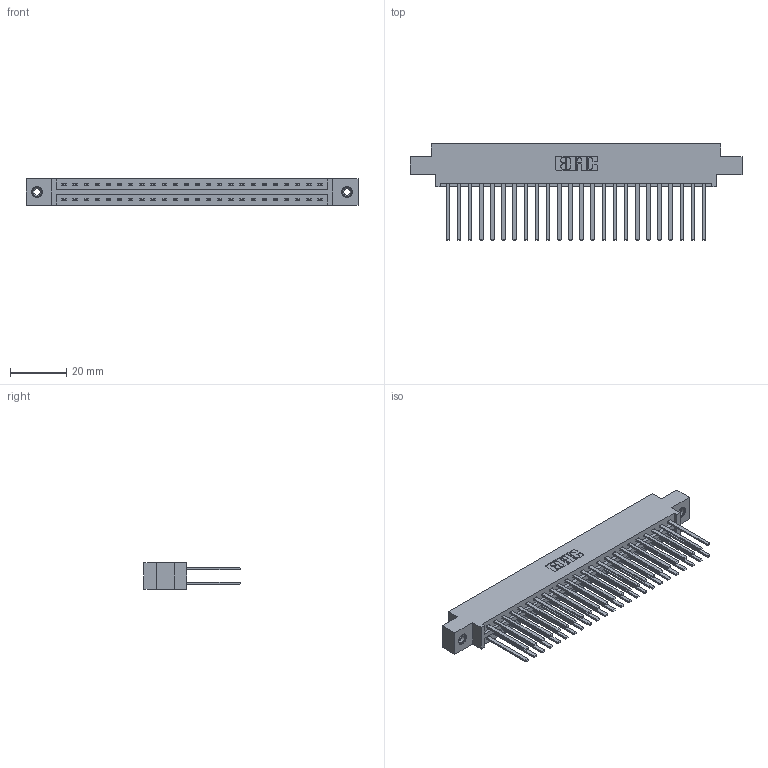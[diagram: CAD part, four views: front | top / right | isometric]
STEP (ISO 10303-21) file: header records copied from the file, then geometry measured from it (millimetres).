
FILE_DESCRIPTION (( 'STEP AP203' ), '1' );
FILE_NAME ('337-048-544-808.STEP', '2019-10-11T15:40:10', ( '' ), ( '' ), 'SwSTEP 2.0', 'SolidWorks 2016', '' );
FILE_SCHEMA (( 'CONFIG_CONTROL_DESIGN' ));
Length unit declared in the file: inch
Products named in the file (4): 345-250-001_345-250-003-102; 337-048-544-808; 337 Part_0.170 Offset - 0.156 Dia-TI; 345-292-001_345-293-144
Assembly tree (51 placements, depth 2):
  337-048-544-808
    337 Part_0.170 Offset - 0.156 Dia-TI
    345-292-001_345-293-144  x48
    345-250-001_345-250-003-102  x2
Bounding box: 118.11 x 34.3 x 9.4 mm (x, y, z)
Volume: 12756.6 mm3; surface area: 16576.4 mm2
Topology: 51 solids, 51 shells, 2482 faces, 7323 edges, 4810 vertices
Faces by surface type: plane 1738, cylinder 728, cone 12, torus 4
Entity records: 22070 total; most frequent: CARTESIAN_POINT 3713, ORIENTED_EDGE 3642, DIRECTION 3219, EDGE_CURVE 1821, VECTOR 1677, LINE 1677, VERTEX_POINT 1208, AXIS2_PLACEMENT_3D 771
